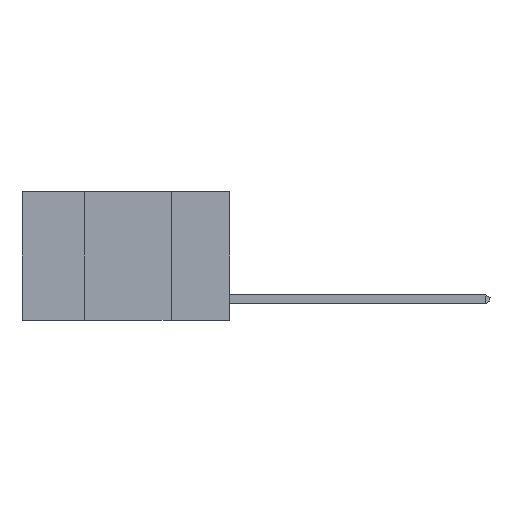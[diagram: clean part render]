
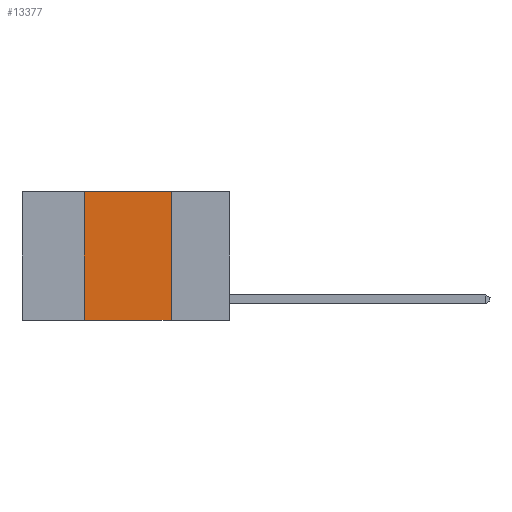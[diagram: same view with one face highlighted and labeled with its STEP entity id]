
A CAD part, left-side view. The second image highlights one B-rep face of the part: STEP entity #13377.
In plain terms, the highlighted planar face has unit normal (-1, 0, 0).
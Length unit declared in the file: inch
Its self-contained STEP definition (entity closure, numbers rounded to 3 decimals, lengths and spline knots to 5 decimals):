
#887 = DIRECTION ( 'NONE',  ( 0., 0., -1. ) ) ;
#2299 = VECTOR ( 'NONE', #19159, 39.37008 ) ;
#3297 = EDGE_LOOP ( 'NONE', ( #14123, #10002, #12087, #6545 ) ) ;
#4484 = DIRECTION ( 'NONE',  ( 0., -1., 0. ) ) ;
#5374 = VERTEX_POINT ( 'NONE', #13453 ) ;
#6227 = LINE ( 'NONE', #17219, #6529 ) ;
#6271 = LINE ( 'NONE', #15415, #2299 ) ;
#6529 = VECTOR ( 'NONE', #4484, 39.37008 ) ;
#6545 = ORIENTED_EDGE ( 'NONE', *, *, #19077, .T. ) ;
#7499 = VERTEX_POINT ( 'NONE', #8212 ) ;
#7583 = VERTEX_POINT ( 'NONE', #14046 ) ;
#8212 = CARTESIAN_POINT ( 'NONE',  ( 0., 0.17, -0.37 ) ) ;
#8957 = VERTEX_POINT ( 'NONE', #21382 ) ;
#9491 = DIRECTION ( 'NONE',  ( 0., 0., -1. ) ) ;
#9504 = CARTESIAN_POINT ( 'NONE',  ( 0., 0.17, 0. ) ) ;
#9946 = PLANE ( 'NONE',  #20495 ) ;
#10002 = ORIENTED_EDGE ( 'NONE', *, *, #13053, .F. ) ;
#11483 = FACE_OUTER_BOUND ( 'NONE', #3297, .T. ) ;
#11623 = LINE ( 'NONE', #9504, #14333 ) ;
#12087 = ORIENTED_EDGE ( 'NONE', *, *, #19677, .F. ) ;
#13053 = EDGE_CURVE ( 'NONE', #5374, #8957, #6227, .T. ) ;
#13377 = ADVANCED_FACE ( 'NONE', ( #11483 ), #9946, .F. ) ;
#13453 = CARTESIAN_POINT ( 'NONE',  ( 0., 0.42, 0. ) ) ;
#14046 = CARTESIAN_POINT ( 'NONE',  ( 0., 0.42, -0.37 ) ) ;
#14123 = ORIENTED_EDGE ( 'NONE', *, *, #18219, .F. ) ;
#14333 = VECTOR ( 'NONE', #887, 39.37008 ) ;
#15155 = VECTOR ( 'NONE', #16595, 39.37008 ) ;
#15415 = CARTESIAN_POINT ( 'NONE',  ( 0., 0.6, -0.37 ) ) ;
#16595 = DIRECTION ( 'NONE',  ( 0., 0., 1. ) ) ;
#17219 = CARTESIAN_POINT ( 'NONE',  ( 0., 0.6, 0. ) ) ;
#18219 = EDGE_CURVE ( 'NONE', #8957, #7499, #11623, .T. ) ;
#18698 = CARTESIAN_POINT ( 'NONE',  ( 0., 0.6, 0. ) ) ;
#19077 = EDGE_CURVE ( 'NONE', #7583, #7499, #6271, .T. ) ;
#19159 = DIRECTION ( 'NONE',  ( 0., -1., 0. ) ) ;
#19677 = EDGE_CURVE ( 'NONE', #7583, #5374, #22005, .T. ) ;
#20495 = AXIS2_PLACEMENT_3D ( 'NONE', #18698, #22369, #9491 ) ;
#21382 = CARTESIAN_POINT ( 'NONE',  ( 0., 0.17, 0. ) ) ;
#22005 = LINE ( 'NONE', #22235, #15155 ) ;
#22235 = CARTESIAN_POINT ( 'NONE',  ( 0., 0.42, 0. ) ) ;
#22369 = DIRECTION ( 'NONE',  ( 1., 0., 0. ) ) ;
